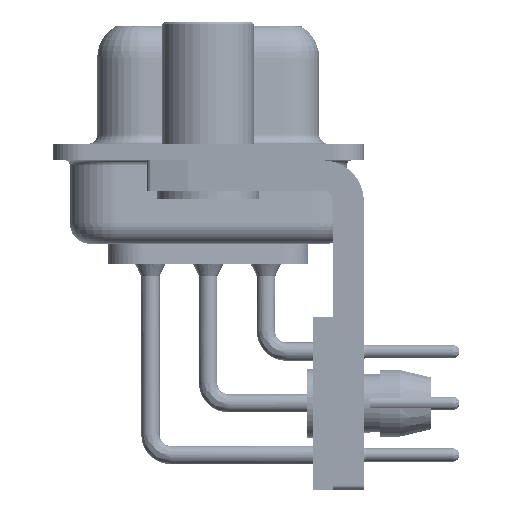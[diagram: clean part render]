
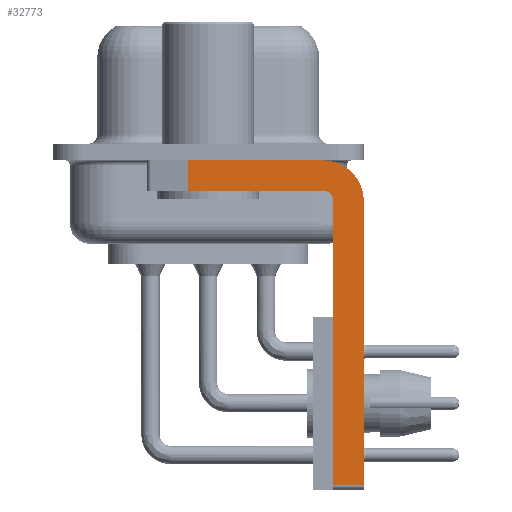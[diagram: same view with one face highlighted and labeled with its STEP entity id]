
A CAD part, left-side view. The second image highlights one B-rep face of the part: STEP entity #32773.
In plain terms, the highlighted planar face has unit normal (-1, 0, 0).
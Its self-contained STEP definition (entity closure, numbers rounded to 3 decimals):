
#143 = VECTOR ( 'NONE', #39386, 1000. ) ;
#674 = LINE ( 'NONE', #11571, #8044 ) ;
#1705 = LINE ( 'NONE', #24356, #9035 ) ;
#1773 = CARTESIAN_POINT ( 'NONE',  ( -2.9, -6.15, -16.35 ) ) ;
#3162 = CARTESIAN_POINT ( 'NONE',  ( -2.9, 0.978, -0.4 ) ) ;
#3911 = ORIENTED_EDGE ( 'NONE', *, *, #40387, .F. ) ;
#4716 = CARTESIAN_POINT ( 'NONE',  ( -2.9, -5.65, -0.4 ) ) ;
#5630 = ORIENTED_EDGE ( 'NONE', *, *, #13943, .T. ) ;
#5941 = CARTESIAN_POINT ( 'NONE',  ( -2.9, -6.15, -16.6 ) ) ;
#6213 = EDGE_CURVE ( 'NONE', #17582, #20068, #32564, .T. ) ;
#6464 = DIRECTION ( 'NONE',  ( 0., 0., -1. ) ) ;
#8044 = VECTOR ( 'NONE', #37026, 1000. ) ;
#8693 = DIRECTION ( 'NONE',  ( 0., 1., 0. ) ) ;
#8716 = CARTESIAN_POINT ( 'NONE',  ( -2.9, -7.65, -2.4 ) ) ;
#9035 = VECTOR ( 'NONE', #8693, 1000. ) ;
#9820 = CARTESIAN_POINT ( 'NONE',  ( -2.9, 3., -0.4 ) ) ;
#11571 = CARTESIAN_POINT ( 'NONE',  ( -2.9, 0.978, -1.9 ) ) ;
#12268 = EDGE_CURVE ( 'NONE', #31687, #26609, #1705, .T. ) ;
#12564 = EDGE_CURVE ( 'NONE', #16272, #31687, #34785, .T. ) ;
#12661 = DIRECTION ( 'NONE',  ( 1., 0., 0. ) ) ;
#13943 = EDGE_CURVE ( 'NONE', #20316, #22077, #32777, .T. ) ;
#15449 = VECTOR ( 'NONE', #39101, 1000. ) ;
#15838 = VECTOR ( 'NONE', #35016, 1000. ) ;
#16272 = VERTEX_POINT ( 'NONE', #36705 ) ;
#16545 = ORIENTED_EDGE ( 'NONE', *, *, #12564, .F. ) ;
#16652 = CARTESIAN_POINT ( 'NONE',  ( -2.9, -5.65, -2.4 ) ) ;
#17404 = AXIS2_PLACEMENT_3D ( 'NONE', #31654, #25309, #6464 ) ;
#17582 = VERTEX_POINT ( 'NONE', #4716 ) ;
#17860 = EDGE_CURVE ( 'NONE', #20316, #16272, #30586, .T. ) ;
#18613 = DIRECTION ( 'NONE',  ( 0., 0., 1. ) ) ;
#19820 = DIRECTION ( 'NONE',  ( 0., 0., 1. ) ) ;
#19919 = CARTESIAN_POINT ( 'NONE',  ( -2.9, -7.65, -2.4 ) ) ;
#20068 = VERTEX_POINT ( 'NONE', #8716 ) ;
#20079 = AXIS2_PLACEMENT_3D ( 'NONE', #31626, #12661, #34795 ) ;
#20316 = VERTEX_POINT ( 'NONE', #1773 ) ;
#20332 = CARTESIAN_POINT ( 'NONE',  ( -2.9, -5.65, -16.35 ) ) ;
#20568 = CARTESIAN_POINT ( 'NONE',  ( -2.9, -7.65, -16.35 ) ) ;
#21634 = EDGE_CURVE ( 'NONE', #40134, #26609, #674, .T. ) ;
#22068 = VECTOR ( 'NONE', #18613, 1000. ) ;
#22077 = VERTEX_POINT ( 'NONE', #20568 ) ;
#23133 = CARTESIAN_POINT ( 'NONE',  ( -2.9, 0.978, -1.9 ) ) ;
#24356 = CARTESIAN_POINT ( 'NONE',  ( -2.9, -5.65, -1.9 ) ) ;
#25309 = DIRECTION ( 'NONE',  ( 1., 0., 0. ) ) ;
#25376 = EDGE_CURVE ( 'NONE', #40134, #17582, #26169, .T. ) ;
#25786 = LINE ( 'NONE', #19919, #15449 ) ;
#26169 = LINE ( 'NONE', #9820, #15838 ) ;
#26414 = ORIENTED_EDGE ( 'NONE', *, *, #21634, .T. ) ;
#26609 = VERTEX_POINT ( 'NONE', #23133 ) ;
#30342 = ORIENTED_EDGE ( 'NONE', *, *, #17860, .F. ) ;
#30586 = LINE ( 'NONE', #5941, #22068 ) ;
#31626 = CARTESIAN_POINT ( 'NONE',  ( -2.9, -5.65, -2.4 ) ) ;
#31654 = CARTESIAN_POINT ( 'NONE',  ( -2.9, -5.65, -2.4 ) ) ;
#31687 = VERTEX_POINT ( 'NONE', #37025 ) ;
#31747 = EDGE_LOOP ( 'NONE', ( #34215, #26414, #33093, #16545, #30342, #5630, #3911, #38091 ) ) ;
#32564 = CIRCLE ( 'NONE', #20079, 2. ) ;
#32773 = ADVANCED_FACE ( 'NONE', ( #39411 ), #38034, .F. ) ;
#32777 = LINE ( 'NONE', #20332, #143 ) ;
#33093 = ORIENTED_EDGE ( 'NONE', *, *, #12268, .F. ) ;
#34215 = ORIENTED_EDGE ( 'NONE', *, *, #25376, .F. ) ;
#34785 = CIRCLE ( 'NONE', #38411, 0.5 ) ;
#34795 = DIRECTION ( 'NONE',  ( 0., 0., -1. ) ) ;
#35016 = DIRECTION ( 'NONE',  ( 0., -1., 0. ) ) ;
#36705 = CARTESIAN_POINT ( 'NONE',  ( -2.9, -6.15, -2.4 ) ) ;
#37025 = CARTESIAN_POINT ( 'NONE',  ( -2.9, -5.65, -1.9 ) ) ;
#37026 = DIRECTION ( 'NONE',  ( 0., 0., -1. ) ) ;
#38034 = PLANE ( 'NONE',  #17404 ) ;
#38091 = ORIENTED_EDGE ( 'NONE', *, *, #6213, .F. ) ;
#38411 = AXIS2_PLACEMENT_3D ( 'NONE', #16652, #38859, #19820 ) ;
#38859 = DIRECTION ( 'NONE',  ( -1., 0., 0. ) ) ;
#39101 = DIRECTION ( 'NONE',  ( 0., 0., -1. ) ) ;
#39386 = DIRECTION ( 'NONE',  ( 0., -1., 0. ) ) ;
#39411 = FACE_OUTER_BOUND ( 'NONE', #31747, .T. ) ;
#40134 = VERTEX_POINT ( 'NONE', #3162 ) ;
#40387 = EDGE_CURVE ( 'NONE', #20068, #22077, #25786, .T. ) ;
